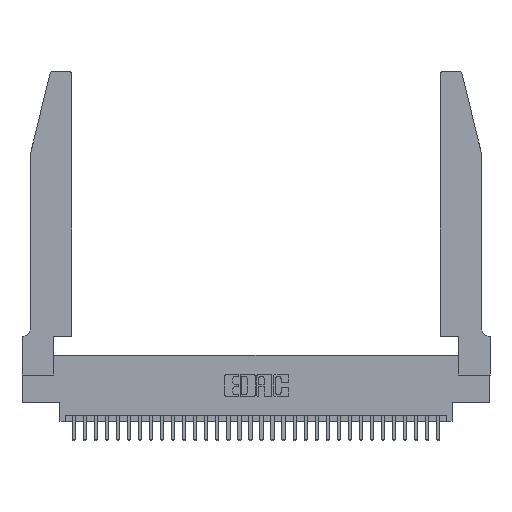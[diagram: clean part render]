
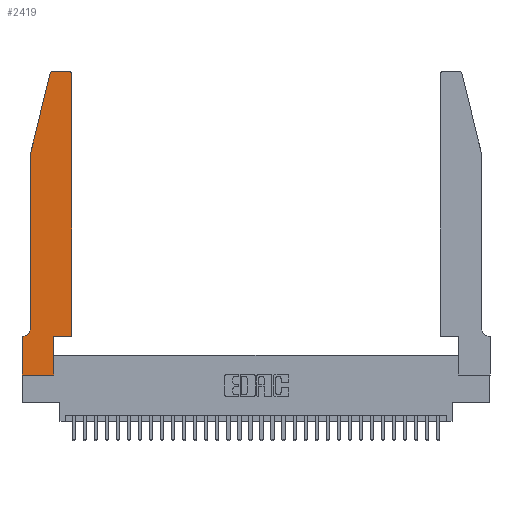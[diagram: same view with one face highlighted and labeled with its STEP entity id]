
A CAD part, top view. The second image highlights one B-rep face of the part: STEP entity #2419.
In plain terms, the highlighted planar face has unit normal (0, 0, 1).
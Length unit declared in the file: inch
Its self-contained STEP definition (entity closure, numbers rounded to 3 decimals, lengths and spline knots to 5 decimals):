
#280 = VERTEX_POINT ( 'NONE', #21591 ) ;
#460 = VERTEX_POINT ( 'NONE', #30156 ) ;
#477 = VERTEX_POINT ( 'NONE', #29933 ) ;
#627 = VECTOR ( 'NONE', #5653, 39.37008 ) ;
#1906 = EDGE_CURVE ( 'NONE', #31286, #477, #4086, .T. ) ;
#1936 = VECTOR ( 'NONE', #6131, 39.37008 ) ;
#1949 = DIRECTION ( 'NONE',  ( 0., 0., -1. ) ) ;
#2003 = EDGE_CURVE ( 'NONE', #11768, #17398, #2465, .T. ) ;
#2419 = ADVANCED_FACE ( 'NONE', ( #17560 ), #3488, .T. ) ;
#2465 = CIRCLE ( 'NONE', #17559, 0.03 ) ;
#2723 = DIRECTION ( 'NONE',  ( 0., -1., 0. ) ) ;
#2937 = DIRECTION ( 'NONE',  ( 0., 1., 0. ) ) ;
#3488 = PLANE ( 'NONE',  #27151 ) ;
#3659 = ORIENTED_EDGE ( 'NONE', *, *, #1906, .T. ) ;
#3816 = LINE ( 'NONE', #10658, #29985 ) ;
#4086 = CIRCLE ( 'NONE', #9081, 0.03 ) ;
#4452 = DIRECTION ( 'NONE',  ( 1., 0., 0. ) ) ;
#5243 = DIRECTION ( 'NONE',  ( 1., 0., 0. ) ) ;
#5653 = DIRECTION ( 'NONE',  ( 0., 1., 0. ) ) ;
#5996 = DIRECTION ( 'NONE',  ( 1., 0., 0. ) ) ;
#6131 = DIRECTION ( 'NONE',  ( 1., 0., 0. ) ) ;
#6189 = VECTOR ( 'NONE', #16818, 39.37008 ) ;
#6681 = VERTEX_POINT ( 'NONE', #14096 ) ;
#7893 = LINE ( 'NONE', #20869, #20559 ) ;
#8357 = CARTESIAN_POINT ( 'NONE',  ( 0.284, 2.75, 0.37 ) ) ;
#8465 = DIRECTION ( 'NONE',  ( 0., 0., 1. ) ) ;
#9081 = AXIS2_PLACEMENT_3D ( 'NONE', #29846, #29114, #4452 ) ;
#10077 = ORIENTED_EDGE ( 'NONE', *, *, #24127, .T. ) ;
#10329 = CARTESIAN_POINT ( 'NONE',  ( 0.2605, 2.75, 0.37 ) ) ;
#10658 = CARTESIAN_POINT ( 'NONE',  ( 0.4505, 0.35, 0.37 ) ) ;
#11196 = DIRECTION ( 'NONE',  ( 1., 0., 0. ) ) ;
#11323 = CARTESIAN_POINT ( 'NONE',  ( 0., 0., 0.37 ) ) ;
#11758 = VECTOR ( 'NONE', #23949, 39.37008 ) ;
#11766 = CARTESIAN_POINT ( 'NONE',  ( 0., 0., 0.37 ) ) ;
#11768 = VERTEX_POINT ( 'NONE', #29125 ) ;
#12745 = ORIENTED_EDGE ( 'NONE', *, *, #28140, .T. ) ;
#12952 = LINE ( 'NONE', #24492, #6189 ) ;
#13337 = EDGE_CURVE ( 'NONE', #32614, #11768, #3816, .T. ) ;
#13526 = VERTEX_POINT ( 'NONE', #31506 ) ;
#13662 = EDGE_CURVE ( 'NONE', #460, #6681, #12952, .T. ) ;
#13963 = EDGE_CURVE ( 'NONE', #17398, #31286, #17668, .T. ) ;
#14007 = VECTOR ( 'NONE', #5243, 39.37008 ) ;
#14096 = CARTESIAN_POINT ( 'NONE',  ( 0., 0.35, 0.37 ) ) ;
#15397 = ORIENTED_EDGE ( 'NONE', *, *, #2003, .T. ) ;
#15524 = EDGE_LOOP ( 'NONE', ( #24960, #3659, #25216, #19149, #12745, #26880, #20858, #10077, #20333, #19482, #27338, #15397 ) ) ;
#15573 = VERTEX_POINT ( 'NONE', #11766 ) ;
#15873 = DIRECTION ( 'NONE',  ( -0.239, -0.971, 0. ) ) ;
#16818 = DIRECTION ( 'NONE',  ( -1., 0., 0. ) ) ;
#17203 = CARTESIAN_POINT ( 'NONE',  ( 0.0055, 0.42, 0.37 ) ) ;
#17398 = VERTEX_POINT ( 'NONE', #22176 ) ;
#17434 = CARTESIAN_POINT ( 'NONE',  ( 0.4505, 0.35, 0.37 ) ) ;
#17559 = AXIS2_PLACEMENT_3D ( 'NONE', #21436, #8465, #5996 ) ;
#17560 = FACE_OUTER_BOUND ( 'NONE', #15524, .T. ) ;
#17668 = LINE ( 'NONE', #10329, #23643 ) ;
#18331 = CARTESIAN_POINT ( 'NONE',  ( 0.2865, 0.35, 0.37 ) ) ;
#18475 = LINE ( 'NONE', #11323, #11758 ) ;
#18900 = VECTOR ( 'NONE', #2723, 39.37008 ) ;
#19149 = ORIENTED_EDGE ( 'NONE', *, *, #31517, .T. ) ;
#19482 = ORIENTED_EDGE ( 'NONE', *, *, #22001, .T. ) ;
#19680 = VERTEX_POINT ( 'NONE', #29136 ) ;
#19728 = DIRECTION ( 'NONE',  ( -1., 0., 0. ) ) ;
#20333 = ORIENTED_EDGE ( 'NONE', *, *, #31249, .T. ) ;
#20559 = VECTOR ( 'NONE', #15873, 39.37008 ) ;
#20719 = LINE ( 'NONE', #27904, #14007 ) ;
#20858 = ORIENTED_EDGE ( 'NONE', *, *, #31760, .T. ) ;
#20869 = CARTESIAN_POINT ( 'NONE',  ( 0.0755, 2., 0.37 ) ) ;
#20887 = LINE ( 'NONE', #18331, #627 ) ;
#21346 = CARTESIAN_POINT ( 'NONE',  ( 0., 0., 0.37 ) ) ;
#21436 = CARTESIAN_POINT ( 'NONE',  ( 0.4205, 2.72, 0.37 ) ) ;
#21591 = CARTESIAN_POINT ( 'NONE',  ( 0.0755, 2., 0.37 ) ) ;
#21664 = CARTESIAN_POINT ( 'NONE',  ( 0.2865, 0.35, 0.37 ) ) ;
#22001 = EDGE_CURVE ( 'NONE', #26132, #32614, #20719, .T. ) ;
#22176 = CARTESIAN_POINT ( 'NONE',  ( 0.4205, 2.75, 0.37 ) ) ;
#23069 = CARTESIAN_POINT ( 'NONE',  ( 0.0755, 2., 0.37 ) ) ;
#23643 = VECTOR ( 'NONE', #28032, 39.37008 ) ;
#23949 = DIRECTION ( 'NONE',  ( 0., -1., 0. ) ) ;
#24127 = EDGE_CURVE ( 'NONE', #15573, #13526, #28181, .T. ) ;
#24492 = CARTESIAN_POINT ( 'NONE',  ( 0.0755, 0.35, 0.37 ) ) ;
#24960 = ORIENTED_EDGE ( 'NONE', *, *, #13963, .T. ) ;
#25216 = ORIENTED_EDGE ( 'NONE', *, *, #29409, .T. ) ;
#26132 = VERTEX_POINT ( 'NONE', #21664 ) ;
#26390 = DIRECTION ( 'NONE',  ( 0., 0., 1. ) ) ;
#26880 = ORIENTED_EDGE ( 'NONE', *, *, #13662, .T. ) ;
#27151 = AXIS2_PLACEMENT_3D ( 'NONE', #31288, #26390, #11196 ) ;
#27338 = ORIENTED_EDGE ( 'NONE', *, *, #13337, .T. ) ;
#27904 = CARTESIAN_POINT ( 'NONE',  ( 0.4505, 0.35, 0.37 ) ) ;
#28032 = DIRECTION ( 'NONE',  ( -1., 0., 0. ) ) ;
#28140 = EDGE_CURVE ( 'NONE', #19680, #460, #29108, .T. ) ;
#28181 = LINE ( 'NONE', #21346, #1936 ) ;
#29108 = CIRCLE ( 'NONE', #29286, 0.07 ) ;
#29114 = DIRECTION ( 'NONE',  ( 0., 0., 1. ) ) ;
#29125 = CARTESIAN_POINT ( 'NONE',  ( 0.4505, 2.72, 0.37 ) ) ;
#29136 = CARTESIAN_POINT ( 'NONE',  ( 0.0755, 0.42, 0.37 ) ) ;
#29286 = AXIS2_PLACEMENT_3D ( 'NONE', #17203, #1949, #19728 ) ;
#29409 = EDGE_CURVE ( 'NONE', #477, #280, #7893, .T. ) ;
#29846 = CARTESIAN_POINT ( 'NONE',  ( 0.284, 2.72, 0.37 ) ) ;
#29933 = CARTESIAN_POINT ( 'NONE',  ( 0.25487, 2.72718, 0.37 ) ) ;
#29985 = VECTOR ( 'NONE', #2937, 39.37008 ) ;
#30156 = CARTESIAN_POINT ( 'NONE',  ( 0.0055, 0.35, 0.37 ) ) ;
#31249 = EDGE_CURVE ( 'NONE', #13526, #26132, #20887, .T. ) ;
#31286 = VERTEX_POINT ( 'NONE', #8357 ) ;
#31288 = CARTESIAN_POINT ( 'NONE',  ( 0., 0.35, 0.37 ) ) ;
#31506 = CARTESIAN_POINT ( 'NONE',  ( 0.2865, 0., 0.37 ) ) ;
#31517 = EDGE_CURVE ( 'NONE', #280, #19680, #32303, .T. ) ;
#31760 = EDGE_CURVE ( 'NONE', #6681, #15573, #18475, .T. ) ;
#32303 = LINE ( 'NONE', #23069, #18900 ) ;
#32614 = VERTEX_POINT ( 'NONE', #17434 ) ;
